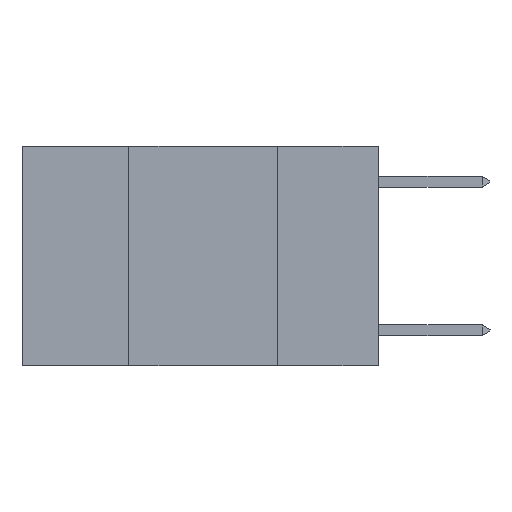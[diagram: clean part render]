
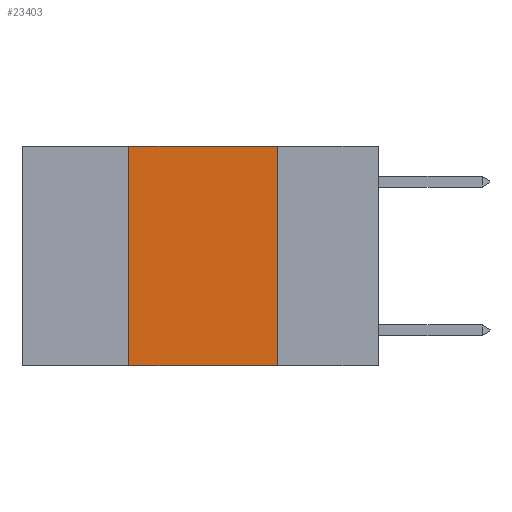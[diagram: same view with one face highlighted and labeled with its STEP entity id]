
A CAD part, left-side view. The second image highlights one B-rep face of the part: STEP entity #23403.
In plain terms, the highlighted planar face has unit normal (-1, 0, 0).
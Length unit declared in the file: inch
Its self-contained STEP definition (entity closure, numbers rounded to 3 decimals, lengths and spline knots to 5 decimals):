
#291 = EDGE_CURVE ( 'NONE', #5489, #11039, #5323, .T. ) ;
#637 = CARTESIAN_POINT ( 'NONE',  ( 0., 0.42, 0. ) ) ;
#953 = CARTESIAN_POINT ( 'NONE',  ( 0., 0.17, 0. ) ) ;
#4527 = DIRECTION ( 'NONE',  ( 0., -1., 0. ) ) ;
#4759 = EDGE_LOOP ( 'NONE', ( #10363, #10577, #10661, #10783 ) ) ;
#4972 = VECTOR ( 'NONE', #23703, 39.37008 ) ;
#5323 = LINE ( 'NONE', #7169, #4972 ) ;
#5489 = VERTEX_POINT ( 'NONE', #6656 ) ;
#5996 = VERTEX_POINT ( 'NONE', #7990 ) ;
#6656 = CARTESIAN_POINT ( 'NONE',  ( 0., 0.42, 0. ) ) ;
#7169 = CARTESIAN_POINT ( 'NONE',  ( 0., 0.6, 0. ) ) ;
#7990 = CARTESIAN_POINT ( 'NONE',  ( 0., 0.17, -0.37 ) ) ;
#9379 = DIRECTION ( 'NONE',  ( 0., 0., -1. ) ) ;
#10363 = ORIENTED_EDGE ( 'NONE', *, *, #13414, .F. ) ;
#10378 = CARTESIAN_POINT ( 'NONE',  ( 0., 0.6, -0.37 ) ) ;
#10577 = ORIENTED_EDGE ( 'NONE', *, *, #291, .F. ) ;
#10661 = ORIENTED_EDGE ( 'NONE', *, *, #12180, .F. ) ;
#10695 = DIRECTION ( 'NONE',  ( 1., 0., 0. ) ) ;
#10783 = ORIENTED_EDGE ( 'NONE', *, *, #10915, .T. ) ;
#10915 = EDGE_CURVE ( 'NONE', #17195, #5996, #20190, .T. ) ;
#11039 = VERTEX_POINT ( 'NONE', #953 ) ;
#12180 = EDGE_CURVE ( 'NONE', #17195, #5489, #24104, .T. ) ;
#13091 = CARTESIAN_POINT ( 'NONE',  ( 0., 0.17, 0. ) ) ;
#13414 = EDGE_CURVE ( 'NONE', #11039, #5996, #13884, .T. ) ;
#13469 = VECTOR ( 'NONE', #9379, 39.37008 ) ;
#13799 = FACE_OUTER_BOUND ( 'NONE', #4759, .T. ) ;
#13884 = LINE ( 'NONE', #13091, #13469 ) ;
#16095 = DIRECTION ( 'NONE',  ( 0., 0., 1. ) ) ;
#17195 = VERTEX_POINT ( 'NONE', #21513 ) ;
#19049 = VECTOR ( 'NONE', #4527, 39.37008 ) ;
#20005 = PLANE ( 'NONE',  #20012 ) ;
#20012 = AXIS2_PLACEMENT_3D ( 'NONE', #21710, #10695, #23385 ) ;
#20190 = LINE ( 'NONE', #10378, #19049 ) ;
#21513 = CARTESIAN_POINT ( 'NONE',  ( 0., 0.42, -0.37 ) ) ;
#21710 = CARTESIAN_POINT ( 'NONE',  ( 0., 0.6, 0. ) ) ;
#23385 = DIRECTION ( 'NONE',  ( 0., 0., -1. ) ) ;
#23403 = ADVANCED_FACE ( 'NONE', ( #13799 ), #20005, .F. ) ;
#23703 = DIRECTION ( 'NONE',  ( 0., -1., 0. ) ) ;
#24056 = VECTOR ( 'NONE', #16095, 39.37008 ) ;
#24104 = LINE ( 'NONE', #637, #24056 ) ;
